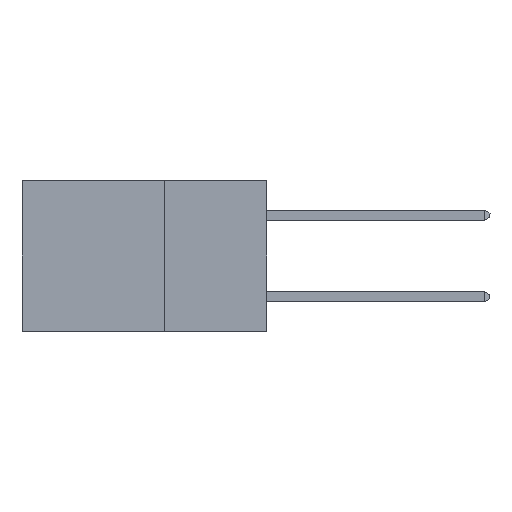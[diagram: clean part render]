
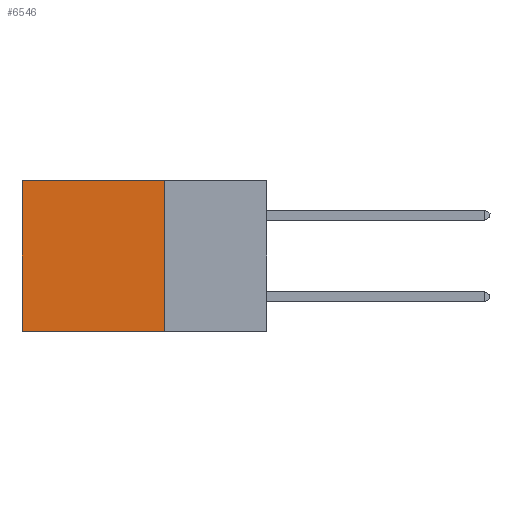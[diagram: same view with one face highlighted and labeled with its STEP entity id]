
A CAD part, left-side view. The second image highlights one B-rep face of the part: STEP entity #6546.
In plain terms, the highlighted planar face has unit normal (-1, 0, 0).
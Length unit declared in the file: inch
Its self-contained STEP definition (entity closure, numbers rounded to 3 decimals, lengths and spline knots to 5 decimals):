
#630 = ORIENTED_EDGE ( 'NONE', *, *, #7971, .T. ) ;
#972 = CARTESIAN_POINT ( 'NONE',  ( 0.2875, 0.25, 0. ) ) ;
#1092 = VERTEX_POINT ( 'NONE', #11502 ) ;
#1107 = CARTESIAN_POINT ( 'NONE',  ( 0.2875, 0.25, -0.37 ) ) ;
#1282 = EDGE_CURVE ( 'NONE', #11678, #6831, #9242, .T. ) ;
#1351 = VECTOR ( 'NONE', #3022, 39.37008 ) ;
#1623 = VECTOR ( 'NONE', #3667, 39.37008 ) ;
#1839 = CARTESIAN_POINT ( 'NONE',  ( 0.2875, 0.25, 0. ) ) ;
#2649 = ORIENTED_EDGE ( 'NONE', *, *, #5641, .T. ) ;
#2676 = CARTESIAN_POINT ( 'NONE',  ( 0.2875, 0.25, 0. ) ) ;
#2820 = DIRECTION ( 'NONE',  ( 0., 0., -1. ) ) ;
#2972 = ORIENTED_EDGE ( 'NONE', *, *, #1282, .F. ) ;
#3022 = DIRECTION ( 'NONE',  ( 0., 0., -1. ) ) ;
#3072 = VECTOR ( 'NONE', #9073, 39.37008 ) ;
#3654 = FACE_OUTER_BOUND ( 'NONE', #11580, .T. ) ;
#3667 = DIRECTION ( 'NONE',  ( 0., 1., 0. ) ) ;
#3769 = LINE ( 'NONE', #1107, #10901 ) ;
#4195 = AXIS2_PLACEMENT_3D ( 'NONE', #1839, #8491, #2820 ) ;
#5599 = LINE ( 'NONE', #6275, #3072 ) ;
#5641 = EDGE_CURVE ( 'NONE', #1092, #9716, #5599, .T. ) ;
#6158 = CARTESIAN_POINT ( 'NONE',  ( 0.2875, 0.6, -0.37 ) ) ;
#6275 = CARTESIAN_POINT ( 'NONE',  ( 0.2875, 0.6, 0. ) ) ;
#6546 = ADVANCED_FACE ( 'NONE', ( #3654 ), #7512, .F. ) ;
#6831 = VERTEX_POINT ( 'NONE', #7954 ) ;
#6901 = DIRECTION ( 'NONE',  ( 0., 1., 0. ) ) ;
#7512 = PLANE ( 'NONE',  #4195 ) ;
#7954 = CARTESIAN_POINT ( 'NONE',  ( 0.2875, 0.25, -0.37 ) ) ;
#7971 = EDGE_CURVE ( 'NONE', #11678, #1092, #12144, .T. ) ;
#7996 = ORIENTED_EDGE ( 'NONE', *, *, #8244, .F. ) ;
#8244 = EDGE_CURVE ( 'NONE', #6831, #9716, #3769, .T. ) ;
#8491 = DIRECTION ( 'NONE',  ( 1., 0., 0. ) ) ;
#9073 = DIRECTION ( 'NONE',  ( 0., 0., -1. ) ) ;
#9242 = LINE ( 'NONE', #10449, #1351 ) ;
#9716 = VERTEX_POINT ( 'NONE', #6158 ) ;
#10449 = CARTESIAN_POINT ( 'NONE',  ( 0.2875, 0.25, 0. ) ) ;
#10901 = VECTOR ( 'NONE', #6901, 39.37008 ) ;
#11502 = CARTESIAN_POINT ( 'NONE',  ( 0.2875, 0.6, 0. ) ) ;
#11580 = EDGE_LOOP ( 'NONE', ( #2649, #7996, #2972, #630 ) ) ;
#11678 = VERTEX_POINT ( 'NONE', #972 ) ;
#12144 = LINE ( 'NONE', #2676, #1623 ) ;
